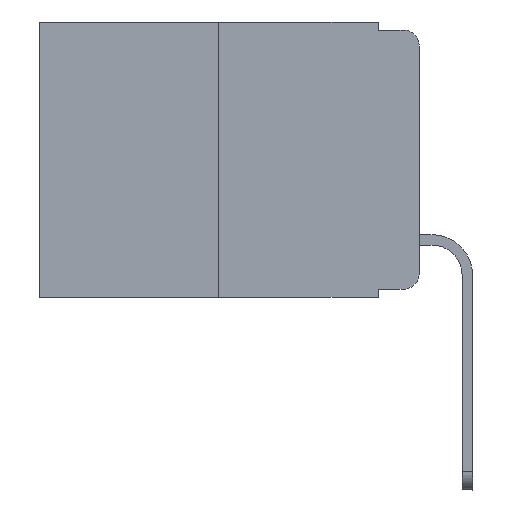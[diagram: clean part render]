
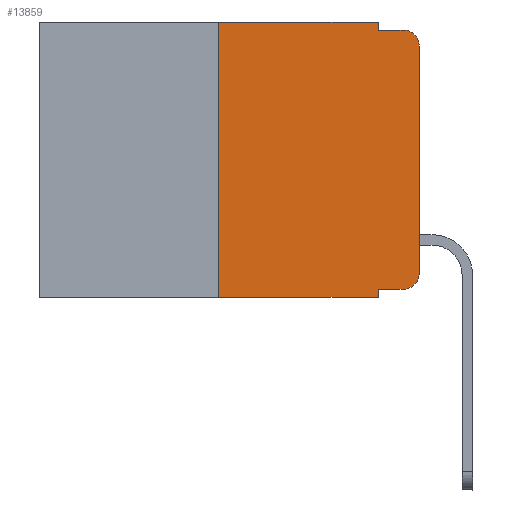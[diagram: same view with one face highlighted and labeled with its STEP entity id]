
A CAD part, left-side view. The second image highlights one B-rep face of the part: STEP entity #13859.
In plain terms, the highlighted planar face has unit normal (-1, 0, 0).
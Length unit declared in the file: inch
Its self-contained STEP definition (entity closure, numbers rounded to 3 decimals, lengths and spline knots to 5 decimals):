
#186 = DIRECTION ( 'NONE',  ( -1., 0., 0. ) ) ;
#253 = CARTESIAN_POINT ( 'NONE',  ( 0., 0.02, -0.03 ) ) ;
#732 = LINE ( 'NONE', #1845, #11407 ) ;
#954 = VERTEX_POINT ( 'NONE', #1690 ) ;
#1101 = EDGE_CURVE ( 'NONE', #3259, #6376, #8871, .T. ) ;
#1126 = EDGE_LOOP ( 'NONE', ( #7153, #10180, #13080, #8755, #2240, #13322, #6295, #9163, #13927, #8341 ) ) ;
#1292 = AXIS2_PLACEMENT_3D ( 'NONE', #14250, #13278, #8690 ) ;
#1690 = CARTESIAN_POINT ( 'NONE',  ( 0., 0.25, 0. ) ) ;
#1845 = CARTESIAN_POINT ( 'NONE',  ( 0., 0.051, 0. ) ) ;
#2240 = ORIENTED_EDGE ( 'NONE', *, *, #4546, .F. ) ;
#2439 = DIRECTION ( 'NONE',  ( 0., 0., 1. ) ) ;
#2801 = CARTESIAN_POINT ( 'NONE',  ( 0., 0.25, -0.343 ) ) ;
#2809 = DIRECTION ( 'NONE',  ( 0., 0., -1. ) ) ;
#2817 = DIRECTION ( 'NONE',  ( 0., -1., 0. ) ) ;
#3259 = VERTEX_POINT ( 'NONE', #2801 ) ;
#3411 = CARTESIAN_POINT ( 'NONE',  ( 0., 0.02, -0.01 ) ) ;
#3470 = FACE_OUTER_BOUND ( 'NONE', #1126, .T. ) ;
#3514 = CARTESIAN_POINT ( 'NONE',  ( 0., 0., -0.03 ) ) ;
#3541 = DIRECTION ( 'NONE',  ( 1., 0., 0. ) ) ;
#4350 = LINE ( 'NONE', #13177, #8340 ) ;
#4354 = AXIS2_PLACEMENT_3D ( 'NONE', #13626, #3541, #8057 ) ;
#4501 = DIRECTION ( 'NONE',  ( 0., -1., 0. ) ) ;
#4546 = EDGE_CURVE ( 'NONE', #954, #11486, #8381, .T. ) ;
#4557 = CARTESIAN_POINT ( 'NONE',  ( 0., 0.051, -0.01 ) ) ;
#4602 = CIRCLE ( 'NONE', #1292, 0.02 ) ;
#4649 = PLANE ( 'NONE',  #4354 ) ;
#4732 = EDGE_CURVE ( 'NONE', #11486, #10741, #9756, .T. ) ;
#4938 = VECTOR ( 'NONE', #2817, 39.37008 ) ;
#4958 = CARTESIAN_POINT ( 'NONE',  ( 0., 0.051, -0.343 ) ) ;
#5253 = CARTESIAN_POINT ( 'NONE',  ( 0., 0.473, -0.343 ) ) ;
#6166 = CARTESIAN_POINT ( 'NONE',  ( 0., 0., -0.313 ) ) ;
#6295 = ORIENTED_EDGE ( 'NONE', *, *, #1101, .T. ) ;
#6376 = VERTEX_POINT ( 'NONE', #4958 ) ;
#6418 = EDGE_CURVE ( 'NONE', #13388, #6376, #732, .T. ) ;
#6499 = EDGE_CURVE ( 'NONE', #13388, #13886, #4350, .T. ) ;
#6811 = LINE ( 'NONE', #7829, #13276 ) ;
#6970 = AXIS2_PLACEMENT_3D ( 'NONE', #253, #186, #13514 ) ;
#7153 = ORIENTED_EDGE ( 'NONE', *, *, #10875, .T. ) ;
#7403 = DIRECTION ( 'NONE',  ( 0., -1., 0. ) ) ;
#7551 = EDGE_CURVE ( 'NONE', #8855, #7989, #8852, .T. ) ;
#7829 = CARTESIAN_POINT ( 'NONE',  ( 0., 0.051, -0.01 ) ) ;
#7958 = VECTOR ( 'NONE', #8490, 39.37008 ) ;
#7962 = EDGE_CURVE ( 'NONE', #3259, #954, #13497, .T. ) ;
#7989 = VERTEX_POINT ( 'NONE', #3411 ) ;
#8057 = DIRECTION ( 'NONE',  ( 0., 0., -1. ) ) ;
#8337 = CARTESIAN_POINT ( 'NONE',  ( 0., 0., 0. ) ) ;
#8340 = VECTOR ( 'NONE', #8725, 39.37008 ) ;
#8341 = ORIENTED_EDGE ( 'NONE', *, *, #12775, .T. ) ;
#8381 = LINE ( 'NONE', #12816, #4938 ) ;
#8490 = DIRECTION ( 'NONE',  ( 0., 0., 1. ) ) ;
#8690 = DIRECTION ( 'NONE',  ( 0., 0., -1. ) ) ;
#8725 = DIRECTION ( 'NONE',  ( 0., -1., 0. ) ) ;
#8755 = ORIENTED_EDGE ( 'NONE', *, *, #4732, .F. ) ;
#8762 = VECTOR ( 'NONE', #12963, 39.37008 ) ;
#8852 = CIRCLE ( 'NONE', #6970, 0.02 ) ;
#8855 = VERTEX_POINT ( 'NONE', #3514 ) ;
#8871 = LINE ( 'NONE', #5253, #10729 ) ;
#9163 = ORIENTED_EDGE ( 'NONE', *, *, #6418, .F. ) ;
#9488 = CARTESIAN_POINT ( 'NONE',  ( 0., 0.051, 0. ) ) ;
#9756 = LINE ( 'NONE', #10991, #8762 ) ;
#10180 = ORIENTED_EDGE ( 'NONE', *, *, #7551, .T. ) ;
#10346 = CARTESIAN_POINT ( 'NONE',  ( 0., 0.25, 0. ) ) ;
#10729 = VECTOR ( 'NONE', #7403, 39.37008 ) ;
#10741 = VERTEX_POINT ( 'NONE', #4557 ) ;
#10875 = EDGE_CURVE ( 'NONE', #11406, #8855, #14119, .T. ) ;
#10991 = CARTESIAN_POINT ( 'NONE',  ( 0., 0.051, 0. ) ) ;
#11406 = VERTEX_POINT ( 'NONE', #6166 ) ;
#11407 = VECTOR ( 'NONE', #2809, 39.37008 ) ;
#11486 = VERTEX_POINT ( 'NONE', #9488 ) ;
#11612 = CARTESIAN_POINT ( 'NONE',  ( 0., 0.02, -0.333 ) ) ;
#12066 = VECTOR ( 'NONE', #2439, 39.37008 ) ;
#12775 = EDGE_CURVE ( 'NONE', #13886, #11406, #4602, .T. ) ;
#12816 = CARTESIAN_POINT ( 'NONE',  ( 0., 0.473, 0. ) ) ;
#12963 = DIRECTION ( 'NONE',  ( 0., 0., -1. ) ) ;
#13080 = ORIENTED_EDGE ( 'NONE', *, *, #13825, .F. ) ;
#13177 = CARTESIAN_POINT ( 'NONE',  ( 0., 0.051, -0.333 ) ) ;
#13276 = VECTOR ( 'NONE', #4501, 39.37008 ) ;
#13278 = DIRECTION ( 'NONE',  ( -1., 0., 0. ) ) ;
#13322 = ORIENTED_EDGE ( 'NONE', *, *, #7962, .F. ) ;
#13388 = VERTEX_POINT ( 'NONE', #13566 ) ;
#13497 = LINE ( 'NONE', #10346, #12066 ) ;
#13514 = DIRECTION ( 'NONE',  ( 0., 0., -1. ) ) ;
#13566 = CARTESIAN_POINT ( 'NONE',  ( 0., 0.051, -0.333 ) ) ;
#13626 = CARTESIAN_POINT ( 'NONE',  ( 0., 0.473, 0. ) ) ;
#13825 = EDGE_CURVE ( 'NONE', #10741, #7989, #6811, .T. ) ;
#13859 = ADVANCED_FACE ( 'NONE', ( #3470 ), #4649, .F. ) ;
#13886 = VERTEX_POINT ( 'NONE', #11612 ) ;
#13927 = ORIENTED_EDGE ( 'NONE', *, *, #6499, .T. ) ;
#14119 = LINE ( 'NONE', #8337, #7958 ) ;
#14250 = CARTESIAN_POINT ( 'NONE',  ( 0., 0.02, -0.313 ) ) ;
